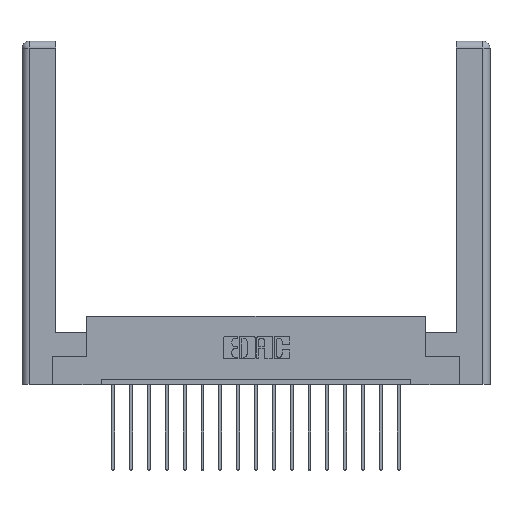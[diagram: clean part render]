
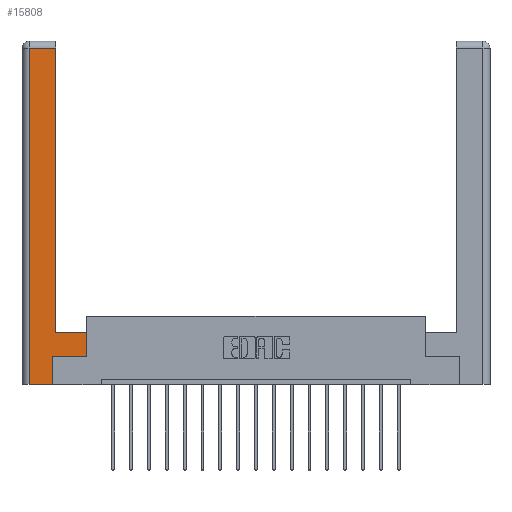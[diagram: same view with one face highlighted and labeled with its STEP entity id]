
A CAD part, top view. The second image highlights one B-rep face of the part: STEP entity #15808.
In plain terms, the highlighted planar face has unit normal (0, 0, 1).
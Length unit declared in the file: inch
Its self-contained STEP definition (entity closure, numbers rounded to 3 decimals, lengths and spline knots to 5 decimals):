
#117 = CARTESIAN_POINT ( 'NONE',  ( 0.0615, 0., 0. ) ) ;
#227 = ORIENTED_EDGE ( 'NONE', *, *, #14105, .T. ) ;
#232 = VECTOR ( 'NONE', #8692, 39.37008 ) ;
#236 = FACE_OUTER_BOUND ( 'NONE', #9514, .T. ) ;
#456 = LINE ( 'NONE', #4746, #7808 ) ;
#746 = DIRECTION ( 'NONE',  ( 0., 1., 0. ) ) ;
#990 = ORIENTED_EDGE ( 'NONE', *, *, #5017, .T. ) ;
#1178 = EDGE_CURVE ( 'NONE', #16999, #12844, #9285, .T. ) ;
#1676 = CARTESIAN_POINT ( 'NONE',  ( 0.565, 0.245, 0. ) ) ;
#2352 = VERTEX_POINT ( 'NONE', #9683 ) ;
#3914 = DIRECTION ( 'NONE',  ( -1., 0., 0. ) ) ;
#4655 = LINE ( 'NONE', #10330, #7101 ) ;
#4746 = CARTESIAN_POINT ( 'NONE',  ( 0.0615, 2.94, 0. ) ) ;
#4923 = CARTESIAN_POINT ( 'NONE',  ( 0.295, 2.94, 0. ) ) ;
#5017 = EDGE_CURVE ( 'NONE', #13597, #15680, #10636, .T. ) ;
#5315 = DIRECTION ( 'NONE',  ( 0., 1., 0. ) ) ;
#6023 = DIRECTION ( 'NONE',  ( -1., 0., 0. ) ) ;
#6327 = AXIS2_PLACEMENT_3D ( 'NONE', #9594, #16936, #3914 ) ;
#7101 = VECTOR ( 'NONE', #6023, 39.37008 ) ;
#7808 = VECTOR ( 'NONE', #14704, 39.37008 ) ;
#7895 = EDGE_CURVE ( 'NONE', #13748, #8722, #12517, .T. ) ;
#8034 = VECTOR ( 'NONE', #13015, 39.37008 ) ;
#8043 = CARTESIAN_POINT ( 'NONE',  ( 0.0615, 0., 0. ) ) ;
#8054 = VECTOR ( 'NONE', #746, 39.37008 ) ;
#8301 = CARTESIAN_POINT ( 'NONE',  ( 0.295, 3., 0. ) ) ;
#8571 = CARTESIAN_POINT ( 'NONE',  ( 0.265, 0., 0. ) ) ;
#8692 = DIRECTION ( 'NONE',  ( 1., 0., 0. ) ) ;
#8722 = VERTEX_POINT ( 'NONE', #8043 ) ;
#8777 = EDGE_CURVE ( 'NONE', #8722, #2352, #15876, .T. ) ;
#9257 = VERTEX_POINT ( 'NONE', #16150 ) ;
#9285 = LINE ( 'NONE', #13825, #18292 ) ;
#9514 = EDGE_LOOP ( 'NONE', ( #990, #15179, #15712, #14026, #12776, #11795, #11196, #227 ) ) ;
#9594 = CARTESIAN_POINT ( 'NONE',  ( 0., 0., 0. ) ) ;
#9683 = CARTESIAN_POINT ( 'NONE',  ( 0.265, 0., 0. ) ) ;
#10118 = CARTESIAN_POINT ( 'NONE',  ( 0.265, 0.245, 0. ) ) ;
#10330 = CARTESIAN_POINT ( 'NONE',  ( 0.295, 0.45, 0. ) ) ;
#10636 = LINE ( 'NONE', #8301, #18508 ) ;
#11029 = CARTESIAN_POINT ( 'NONE',  ( 0.295, 0.45, 0. ) ) ;
#11196 = ORIENTED_EDGE ( 'NONE', *, *, #12879, .T. ) ;
#11795 = ORIENTED_EDGE ( 'NONE', *, *, #1178, .T. ) ;
#11849 = LINE ( 'NONE', #14947, #8054 ) ;
#12517 = LINE ( 'NONE', #117, #14799 ) ;
#12776 = ORIENTED_EDGE ( 'NONE', *, *, #13379, .T. ) ;
#12844 = VERTEX_POINT ( 'NONE', #1676 ) ;
#12879 = EDGE_CURVE ( 'NONE', #12844, #9257, #11849, .T. ) ;
#13015 = DIRECTION ( 'NONE',  ( 0., 1., 0. ) ) ;
#13379 = EDGE_CURVE ( 'NONE', #2352, #16999, #14776, .T. ) ;
#13533 = EDGE_CURVE ( 'NONE', #15680, #13748, #456, .T. ) ;
#13597 = VERTEX_POINT ( 'NONE', #11029 ) ;
#13748 = VERTEX_POINT ( 'NONE', #17157 ) ;
#13825 = CARTESIAN_POINT ( 'NONE',  ( 0.565, 0.245, 0. ) ) ;
#14026 = ORIENTED_EDGE ( 'NONE', *, *, #8777, .T. ) ;
#14105 = EDGE_CURVE ( 'NONE', #9257, #13597, #4655, .T. ) ;
#14704 = DIRECTION ( 'NONE',  ( -1., 0., 0. ) ) ;
#14776 = LINE ( 'NONE', #10118, #8034 ) ;
#14799 = VECTOR ( 'NONE', #15798, 39.37008 ) ;
#14867 = CARTESIAN_POINT ( 'NONE',  ( 0.265, 0.245, 0. ) ) ;
#14947 = CARTESIAN_POINT ( 'NONE',  ( 0.565, 0.45, 0. ) ) ;
#15179 = ORIENTED_EDGE ( 'NONE', *, *, #13533, .T. ) ;
#15273 = DIRECTION ( 'NONE',  ( 1., 0., 0. ) ) ;
#15680 = VERTEX_POINT ( 'NONE', #4923 ) ;
#15712 = ORIENTED_EDGE ( 'NONE', *, *, #7895, .T. ) ;
#15798 = DIRECTION ( 'NONE',  ( 0., -1., 0. ) ) ;
#15808 = ADVANCED_FACE ( 'NONE', ( #236 ), #16753, .F. ) ;
#15876 = LINE ( 'NONE', #8571, #232 ) ;
#16150 = CARTESIAN_POINT ( 'NONE',  ( 0.565, 0.45, 0. ) ) ;
#16753 = PLANE ( 'NONE',  #6327 ) ;
#16936 = DIRECTION ( 'NONE',  ( 0., 0., -1. ) ) ;
#16999 = VERTEX_POINT ( 'NONE', #14867 ) ;
#17157 = CARTESIAN_POINT ( 'NONE',  ( 0.0615, 2.94, 0. ) ) ;
#18292 = VECTOR ( 'NONE', #15273, 39.37008 ) ;
#18508 = VECTOR ( 'NONE', #5315, 39.37008 ) ;
